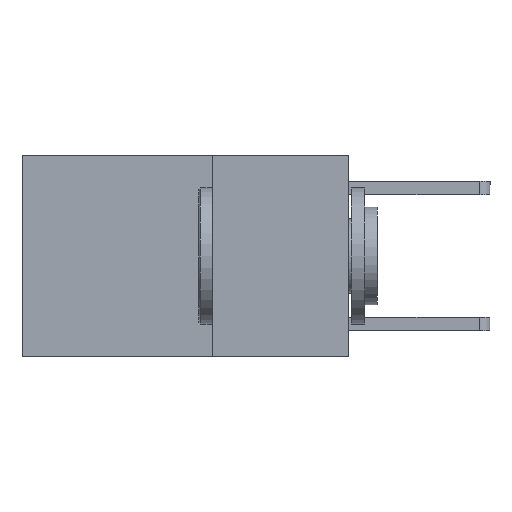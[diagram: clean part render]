
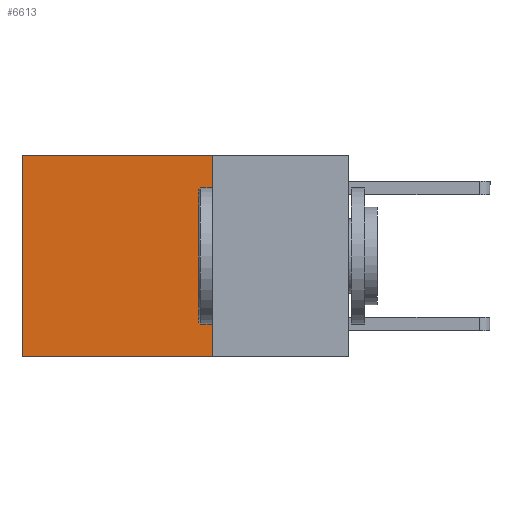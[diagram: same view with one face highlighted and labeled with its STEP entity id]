
A CAD part, left-side view. The second image highlights one B-rep face of the part: STEP entity #6613.
In plain terms, the highlighted planar face has unit normal (-1, 0, 0).
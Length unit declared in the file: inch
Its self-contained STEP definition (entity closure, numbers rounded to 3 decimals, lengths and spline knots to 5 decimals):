
#36 = ORIENTED_EDGE ( 'NONE', *, *, #4997, .F. ) ;
#240 = ORIENTED_EDGE ( 'NONE', *, *, #3648, .T. ) ;
#392 = ORIENTED_EDGE ( 'NONE', *, *, #3836, .T. ) ;
#831 = VECTOR ( 'NONE', #5945, 39.37008 ) ;
#1264 = CARTESIAN_POINT ( 'NONE',  ( 0.2625, 0.25, 0. ) ) ;
#1778 = DIRECTION ( 'NONE',  ( 0., 0., -1. ) ) ;
#1816 = EDGE_CURVE ( 'NONE', #4356, #4761, #4577, .T. ) ;
#1951 = CARTESIAN_POINT ( 'NONE',  ( 0.2625, 0.25, -0.37 ) ) ;
#2824 = VECTOR ( 'NONE', #4885, 39.37008 ) ;
#2913 = VERTEX_POINT ( 'NONE', #7624 ) ;
#2952 = CARTESIAN_POINT ( 'NONE',  ( 0.2625, 0.25, -0.37 ) ) ;
#3040 = VECTOR ( 'NONE', #1778, 39.37008 ) ;
#3207 = ORIENTED_EDGE ( 'NONE', *, *, #1816, .F. ) ;
#3353 = LINE ( 'NONE', #8232, #2824 ) ;
#3366 = FACE_OUTER_BOUND ( 'NONE', #5750, .T. ) ;
#3648 = EDGE_CURVE ( 'NONE', #4356, #8123, #7920, .T. ) ;
#3798 = CARTESIAN_POINT ( 'NONE',  ( 0.2625, 0.25, 0. ) ) ;
#3836 = EDGE_CURVE ( 'NONE', #8123, #2913, #3353, .T. ) ;
#4310 = CARTESIAN_POINT ( 'NONE',  ( 0.2625, 0.6, 0. ) ) ;
#4356 = VERTEX_POINT ( 'NONE', #6124 ) ;
#4577 = LINE ( 'NONE', #5201, #3040 ) ;
#4761 = VERTEX_POINT ( 'NONE', #2952 ) ;
#4885 = DIRECTION ( 'NONE',  ( 0., 0., -1. ) ) ;
#4997 = EDGE_CURVE ( 'NONE', #4761, #2913, #7922, .T. ) ;
#5201 = CARTESIAN_POINT ( 'NONE',  ( 0.2625, 0.25, 0. ) ) ;
#5395 = DIRECTION ( 'NONE',  ( 0., 0., -1. ) ) ;
#5750 = EDGE_LOOP ( 'NONE', ( #392, #36, #3207, #240 ) ) ;
#5945 = DIRECTION ( 'NONE',  ( 0., 1., 0. ) ) ;
#6124 = CARTESIAN_POINT ( 'NONE',  ( 0.2625, 0.25, 0. ) ) ;
#6430 = VECTOR ( 'NONE', #6676, 39.37008 ) ;
#6510 = AXIS2_PLACEMENT_3D ( 'NONE', #1264, #8703, #5395 ) ;
#6613 = ADVANCED_FACE ( 'NONE', ( #3366 ), #7397, .F. ) ;
#6676 = DIRECTION ( 'NONE',  ( 0., 1., 0. ) ) ;
#7397 = PLANE ( 'NONE',  #6510 ) ;
#7624 = CARTESIAN_POINT ( 'NONE',  ( 0.2625, 0.6, -0.37 ) ) ;
#7920 = LINE ( 'NONE', #3798, #831 ) ;
#7922 = LINE ( 'NONE', #1951, #6430 ) ;
#8123 = VERTEX_POINT ( 'NONE', #4310 ) ;
#8232 = CARTESIAN_POINT ( 'NONE',  ( 0.2625, 0.6, 0. ) ) ;
#8703 = DIRECTION ( 'NONE',  ( 1., 0., 0. ) ) ;
